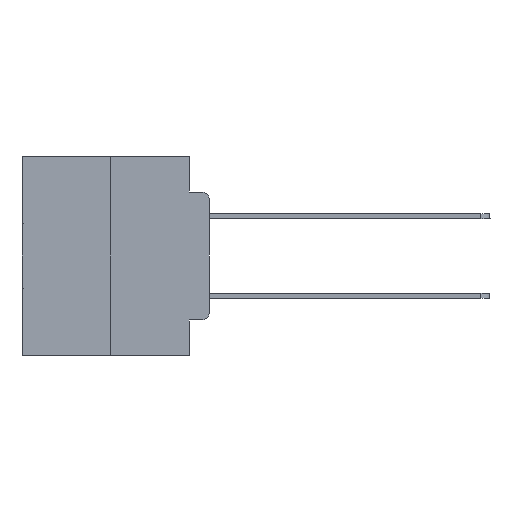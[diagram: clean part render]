
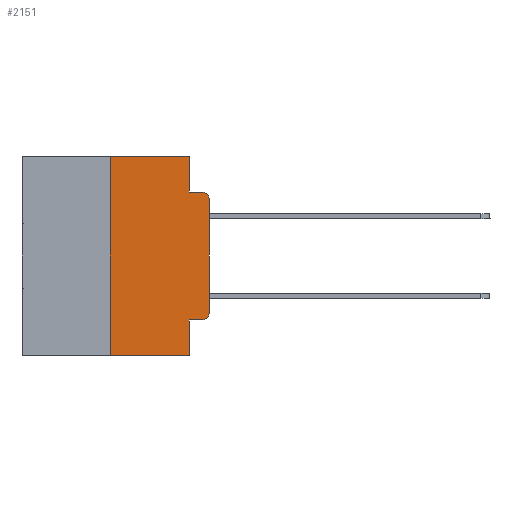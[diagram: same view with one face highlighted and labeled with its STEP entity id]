
A CAD part, left-side view. The second image highlights one B-rep face of the part: STEP entity #2151.
In plain terms, the highlighted planar face has unit normal (-1, 0, 0).
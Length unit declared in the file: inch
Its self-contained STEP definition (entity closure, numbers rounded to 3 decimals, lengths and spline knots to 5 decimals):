
#261 = VECTOR ( 'NONE', #13342, 39.37008 ) ;
#331 = CARTESIAN_POINT ( 'NONE',  ( 0., 0.25, -0.5 ) ) ;
#407 = CIRCLE ( 'NONE', #1795, 0.02 ) ;
#628 = CARTESIAN_POINT ( 'NONE',  ( 0., 0.02, -0.3915 ) ) ;
#954 = VERTEX_POINT ( 'NONE', #331 ) ;
#1109 = VECTOR ( 'NONE', #9002, 39.37008 ) ;
#1795 = AXIS2_PLACEMENT_3D ( 'NONE', #21165, #14210, #21381 ) ;
#1972 = VERTEX_POINT ( 'NONE', #11651 ) ;
#2151 = ADVANCED_FACE ( 'NONE', ( #21931 ), #22369, .F. ) ;
#2445 = CARTESIAN_POINT ( 'NONE',  ( 0., 0.02, -0.4115 ) ) ;
#2588 = ORIENTED_EDGE ( 'NONE', *, *, #4534, .F. ) ;
#2798 = CARTESIAN_POINT ( 'NONE',  ( 0., 0., -0.1085 ) ) ;
#3787 = EDGE_CURVE ( 'NONE', #15285, #18123, #407, .T. ) ;
#4159 = VERTEX_POINT ( 'NONE', #2445 ) ;
#4392 = DIRECTION ( 'NONE',  ( 0., 0., -1. ) ) ;
#4534 = EDGE_CURVE ( 'NONE', #954, #7302, #22715, .T. ) ;
#4658 = ORIENTED_EDGE ( 'NONE', *, *, #24847, .T. ) ;
#5615 = VERTEX_POINT ( 'NONE', #22088 ) ;
#5805 = LINE ( 'NONE', #25666, #13859 ) ;
#6115 = CARTESIAN_POINT ( 'NONE',  ( 0., 0.051, -0.0885 ) ) ;
#6261 = EDGE_CURVE ( 'NONE', #5615, #4159, #24897, .T. ) ;
#6532 = CARTESIAN_POINT ( 'NONE',  ( 0., 0.473, 0. ) ) ;
#7302 = VERTEX_POINT ( 'NONE', #28600 ) ;
#7344 = LINE ( 'NONE', #6532, #1109 ) ;
#7635 = EDGE_LOOP ( 'NONE', ( #19689, #23315, #12401, #9533, #11017, #2588, #18271, #27425, #18506, #4658 ) ) ;
#8189 = VECTOR ( 'NONE', #22927, 39.37008 ) ;
#8255 = DIRECTION ( 'NONE',  ( 0., 0., -1. ) ) ;
#8274 = DIRECTION ( 'NONE',  ( 0., -1., 0. ) ) ;
#8560 = CARTESIAN_POINT ( 'NONE',  ( 0., 0.051, -0.5 ) ) ;
#9002 = DIRECTION ( 'NONE',  ( 0., -1., 0. ) ) ;
#9475 = EDGE_CURVE ( 'NONE', #1972, #15285, #22641, .T. ) ;
#9533 = ORIENTED_EDGE ( 'NONE', *, *, #15685, .F. ) ;
#10841 = VERTEX_POINT ( 'NONE', #22672 ) ;
#11017 = ORIENTED_EDGE ( 'NONE', *, *, #14577, .F. ) ;
#11101 = CIRCLE ( 'NONE', #12306, 0.02 ) ;
#11651 = CARTESIAN_POINT ( 'NONE',  ( 0., 0., -0.3915 ) ) ;
#12306 = AXIS2_PLACEMENT_3D ( 'NONE', #628, #16984, #26288 ) ;
#12375 = LINE ( 'NONE', #19664, #26361 ) ;
#12401 = ORIENTED_EDGE ( 'NONE', *, *, #25197, .F. ) ;
#13150 = EDGE_CURVE ( 'NONE', #954, #16818, #14796, .T. ) ;
#13342 = DIRECTION ( 'NONE',  ( 0., 0., 1. ) ) ;
#13859 = VECTOR ( 'NONE', #4392, 39.37008 ) ;
#14210 = DIRECTION ( 'NONE',  ( -1., 0., 0. ) ) ;
#14577 = EDGE_CURVE ( 'NONE', #7302, #10841, #7344, .T. ) ;
#14796 = LINE ( 'NONE', #20572, #8189 ) ;
#15004 = CARTESIAN_POINT ( 'NONE',  ( 0., 0.02, -0.0885 ) ) ;
#15285 = VERTEX_POINT ( 'NONE', #2798 ) ;
#15541 = AXIS2_PLACEMENT_3D ( 'NONE', #24633, #24528, #26912 ) ;
#15685 = EDGE_CURVE ( 'NONE', #10841, #22302, #5805, .T. ) ;
#16644 = LINE ( 'NONE', #20906, #28773 ) ;
#16818 = VERTEX_POINT ( 'NONE', #8560 ) ;
#16984 = DIRECTION ( 'NONE',  ( -1., 0., 0. ) ) ;
#17652 = DIRECTION ( 'NONE',  ( 0., 0., 1. ) ) ;
#17978 = VECTOR ( 'NONE', #17652, 39.37008 ) ;
#18123 = VERTEX_POINT ( 'NONE', #15004 ) ;
#18271 = ORIENTED_EDGE ( 'NONE', *, *, #13150, .T. ) ;
#18506 = ORIENTED_EDGE ( 'NONE', *, *, #6261, .T. ) ;
#19664 = CARTESIAN_POINT ( 'NONE',  ( 0., 0.051, 0. ) ) ;
#19689 = ORIENTED_EDGE ( 'NONE', *, *, #9475, .T. ) ;
#19795 = VECTOR ( 'NONE', #8274, 39.37008 ) ;
#19884 = CARTESIAN_POINT ( 'NONE',  ( 0., 0.051, -0.4115 ) ) ;
#20572 = CARTESIAN_POINT ( 'NONE',  ( 0., 0.473, -0.5 ) ) ;
#20906 = CARTESIAN_POINT ( 'NONE',  ( 0., 0.051, -0.0885 ) ) ;
#21165 = CARTESIAN_POINT ( 'NONE',  ( 0., 0.02, -0.1085 ) ) ;
#21381 = DIRECTION ( 'NONE',  ( 0., 0., -1. ) ) ;
#21931 = FACE_OUTER_BOUND ( 'NONE', #7635, .T. ) ;
#22088 = CARTESIAN_POINT ( 'NONE',  ( 0., 0.051, -0.4115 ) ) ;
#22302 = VERTEX_POINT ( 'NONE', #6115 ) ;
#22369 = PLANE ( 'NONE',  #15541 ) ;
#22641 = LINE ( 'NONE', #27737, #261 ) ;
#22672 = CARTESIAN_POINT ( 'NONE',  ( 0., 0.051, 0. ) ) ;
#22715 = LINE ( 'NONE', #24611, #17978 ) ;
#22927 = DIRECTION ( 'NONE',  ( 0., -1., 0. ) ) ;
#23315 = ORIENTED_EDGE ( 'NONE', *, *, #3787, .T. ) ;
#24528 = DIRECTION ( 'NONE',  ( 1., 0., 0. ) ) ;
#24611 = CARTESIAN_POINT ( 'NONE',  ( 0., 0.25, 0. ) ) ;
#24633 = CARTESIAN_POINT ( 'NONE',  ( 0., 0.473, 0. ) ) ;
#24847 = EDGE_CURVE ( 'NONE', #4159, #1972, #11101, .T. ) ;
#24897 = LINE ( 'NONE', #19884, #19795 ) ;
#25197 = EDGE_CURVE ( 'NONE', #22302, #18123, #16644, .T. ) ;
#25666 = CARTESIAN_POINT ( 'NONE',  ( 0., 0.051, 0. ) ) ;
#26288 = DIRECTION ( 'NONE',  ( 0., 0., -1. ) ) ;
#26361 = VECTOR ( 'NONE', #8255, 39.37008 ) ;
#26912 = DIRECTION ( 'NONE',  ( 0., 0., -1. ) ) ;
#27425 = ORIENTED_EDGE ( 'NONE', *, *, #28113, .F. ) ;
#27737 = CARTESIAN_POINT ( 'NONE',  ( 0., 0., 0. ) ) ;
#28113 = EDGE_CURVE ( 'NONE', #5615, #16818, #12375, .T. ) ;
#28600 = CARTESIAN_POINT ( 'NONE',  ( 0., 0.25, 0. ) ) ;
#28773 = VECTOR ( 'NONE', #30268, 39.37008 ) ;
#30268 = DIRECTION ( 'NONE',  ( 0., -1., 0. ) ) ;
